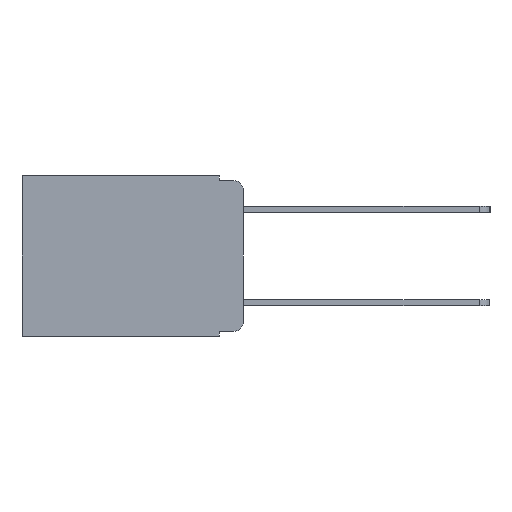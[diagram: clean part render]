
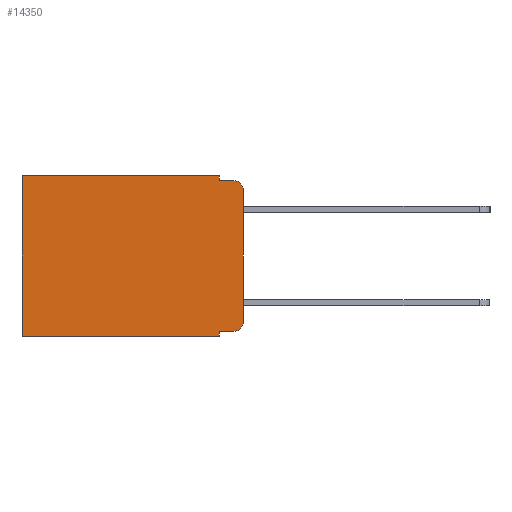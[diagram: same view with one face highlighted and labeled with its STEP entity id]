
A CAD part, left-side view. The second image highlights one B-rep face of the part: STEP entity #14350.
In plain terms, the highlighted planar face has unit normal (-1, 0, 0).
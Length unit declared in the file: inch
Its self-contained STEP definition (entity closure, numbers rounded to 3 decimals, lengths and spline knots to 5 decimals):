
#312 = PLANE ( 'NONE',  #589 ) ;
#418 = CARTESIAN_POINT ( 'NONE',  ( 0.298, 0.051, -0.333 ) ) ;
#589 = AXIS2_PLACEMENT_3D ( 'NONE', #8941, #3991, #15307 ) ;
#1491 = LINE ( 'NONE', #16708, #5077 ) ;
#1650 = CARTESIAN_POINT ( 'NONE',  ( 0.298, 0.02, -0.313 ) ) ;
#2206 = CARTESIAN_POINT ( 'NONE',  ( 0.298, 0.473, 0. ) ) ;
#2486 = EDGE_CURVE ( 'NONE', #20429, #6811, #1491, .T. ) ;
#2555 = EDGE_CURVE ( 'NONE', #3914, #20901, #13183, .T. ) ;
#2796 = ORIENTED_EDGE ( 'NONE', *, *, #11600, .T. ) ;
#2931 = CARTESIAN_POINT ( 'NONE',  ( 0.298, 0.051, -0.343 ) ) ;
#3016 = EDGE_CURVE ( 'NONE', #7371, #6494, #15822, .T. ) ;
#3060 = ORIENTED_EDGE ( 'NONE', *, *, #3016, .T. ) ;
#3174 = DIRECTION ( 'NONE',  ( 0., 0., -1. ) ) ;
#3914 = VERTEX_POINT ( 'NONE', #9957 ) ;
#3938 = CARTESIAN_POINT ( 'NONE',  ( 0.298, 0.02, -0.01 ) ) ;
#3991 = DIRECTION ( 'NONE',  ( 1., 0., 0. ) ) ;
#4057 = DIRECTION ( 'NONE',  ( -1., 0., 0. ) ) ;
#4296 = VECTOR ( 'NONE', #12230, 39.37008 ) ;
#4478 = ORIENTED_EDGE ( 'NONE', *, *, #14993, .T. ) ;
#4531 = VECTOR ( 'NONE', #13227, 39.37008 ) ;
#4848 = LINE ( 'NONE', #2206, #4296 ) ;
#4931 = LINE ( 'NONE', #11329, #7742 ) ;
#5077 = VECTOR ( 'NONE', #18415, 39.37008 ) ;
#5407 = VECTOR ( 'NONE', #17579, 39.37008 ) ;
#6445 = EDGE_CURVE ( 'NONE', #15752, #6494, #4931, .T. ) ;
#6494 = VERTEX_POINT ( 'NONE', #6605 ) ;
#6605 = CARTESIAN_POINT ( 'NONE',  ( 0.298, 0., -0.313 ) ) ;
#6811 = VERTEX_POINT ( 'NONE', #19921 ) ;
#7103 = CARTESIAN_POINT ( 'NONE',  ( 0.298, 0.051, 0. ) ) ;
#7282 = CARTESIAN_POINT ( 'NONE',  ( 0.298, 0.02, -0.333 ) ) ;
#7371 = VERTEX_POINT ( 'NONE', #7282 ) ;
#7706 = EDGE_CURVE ( 'NONE', #15752, #10182, #9283, .T. ) ;
#7742 = VECTOR ( 'NONE', #12919, 39.37008 ) ;
#8877 = CARTESIAN_POINT ( 'NONE',  ( 0.298, 0.051, 0. ) ) ;
#8941 = CARTESIAN_POINT ( 'NONE',  ( 0.298, 0., 0. ) ) ;
#9113 = VECTOR ( 'NONE', #12211, 39.37008 ) ;
#9171 = LINE ( 'NONE', #15173, #16531 ) ;
#9283 = CIRCLE ( 'NONE', #13262, 0.02 ) ;
#9416 = ORIENTED_EDGE ( 'NONE', *, *, #2486, .T. ) ;
#9899 = ORIENTED_EDGE ( 'NONE', *, *, #2555, .F. ) ;
#9957 = CARTESIAN_POINT ( 'NONE',  ( 0.298, 0.051, -0.333 ) ) ;
#10030 = DIRECTION ( 'NONE',  ( -1., 0., 0. ) ) ;
#10182 = VERTEX_POINT ( 'NONE', #3938 ) ;
#10259 = CARTESIAN_POINT ( 'NONE',  ( 0.298, 0.051, -0.01 ) ) ;
#10284 = LINE ( 'NONE', #11360, #5407 ) ;
#11329 = CARTESIAN_POINT ( 'NONE',  ( 0.298, 0., 0. ) ) ;
#11360 = CARTESIAN_POINT ( 'NONE',  ( 0.298, 0.051, 0. ) ) ;
#11600 = EDGE_CURVE ( 'NONE', #3914, #7371, #13858, .T. ) ;
#11615 = VECTOR ( 'NONE', #11850, 39.37008 ) ;
#11756 = FACE_OUTER_BOUND ( 'NONE', #12706, .T. ) ;
#11850 = DIRECTION ( 'NONE',  ( 0., -1., 0. ) ) ;
#12064 = CARTESIAN_POINT ( 'NONE',  ( 0.298, 0., -0.03 ) ) ;
#12211 = DIRECTION ( 'NONE',  ( 0., -1., 0. ) ) ;
#12230 = DIRECTION ( 'NONE',  ( 0., 0., -1. ) ) ;
#12654 = AXIS2_PLACEMENT_3D ( 'NONE', #1650, #4057, #3174 ) ;
#12706 = EDGE_LOOP ( 'NONE', ( #19620, #15092, #17263, #19379, #9416, #4478, #19582, #9899, #2796, #3060 ) ) ;
#12919 = DIRECTION ( 'NONE',  ( 0., 0., -1. ) ) ;
#13183 = LINE ( 'NONE', #8877, #4531 ) ;
#13227 = DIRECTION ( 'NONE',  ( 0., 0., -1. ) ) ;
#13262 = AXIS2_PLACEMENT_3D ( 'NONE', #19299, #10030, #20818 ) ;
#13432 = VERTEX_POINT ( 'NONE', #13726 ) ;
#13726 = CARTESIAN_POINT ( 'NONE',  ( 0.298, 0.473, -0.343 ) ) ;
#13858 = LINE ( 'NONE', #418, #9113 ) ;
#13987 = EDGE_CURVE ( 'NONE', #20429, #15986, #10284, .T. ) ;
#14350 = ADVANCED_FACE ( 'NONE', ( #11756 ), #312, .F. ) ;
#14993 = EDGE_CURVE ( 'NONE', #6811, #13432, #4848, .T. ) ;
#15092 = ORIENTED_EDGE ( 'NONE', *, *, #7706, .T. ) ;
#15173 = CARTESIAN_POINT ( 'NONE',  ( 0.298, 0., -0.343 ) ) ;
#15307 = DIRECTION ( 'NONE',  ( 0., 0., -1. ) ) ;
#15752 = VERTEX_POINT ( 'NONE', #12064 ) ;
#15822 = CIRCLE ( 'NONE', #12654, 0.02 ) ;
#15986 = VERTEX_POINT ( 'NONE', #20325 ) ;
#16432 = EDGE_CURVE ( 'NONE', #20901, #13432, #9171, .T. ) ;
#16531 = VECTOR ( 'NONE', #16717, 39.37008 ) ;
#16708 = CARTESIAN_POINT ( 'NONE',  ( 0.298, 0., 0. ) ) ;
#16717 = DIRECTION ( 'NONE',  ( 0., 1., 0. ) ) ;
#17263 = ORIENTED_EDGE ( 'NONE', *, *, #18903, .F. ) ;
#17579 = DIRECTION ( 'NONE',  ( 0., 0., -1. ) ) ;
#18415 = DIRECTION ( 'NONE',  ( 0., 1., 0. ) ) ;
#18903 = EDGE_CURVE ( 'NONE', #15986, #10182, #19789, .T. ) ;
#19299 = CARTESIAN_POINT ( 'NONE',  ( 0.298, 0.02, -0.03 ) ) ;
#19379 = ORIENTED_EDGE ( 'NONE', *, *, #13987, .F. ) ;
#19582 = ORIENTED_EDGE ( 'NONE', *, *, #16432, .F. ) ;
#19620 = ORIENTED_EDGE ( 'NONE', *, *, #6445, .F. ) ;
#19789 = LINE ( 'NONE', #10259, #11615 ) ;
#19921 = CARTESIAN_POINT ( 'NONE',  ( 0.298, 0.473, 0. ) ) ;
#20325 = CARTESIAN_POINT ( 'NONE',  ( 0.298, 0.051, -0.01 ) ) ;
#20429 = VERTEX_POINT ( 'NONE', #7103 ) ;
#20818 = DIRECTION ( 'NONE',  ( 0., 0., -1. ) ) ;
#20901 = VERTEX_POINT ( 'NONE', #2931 ) ;
